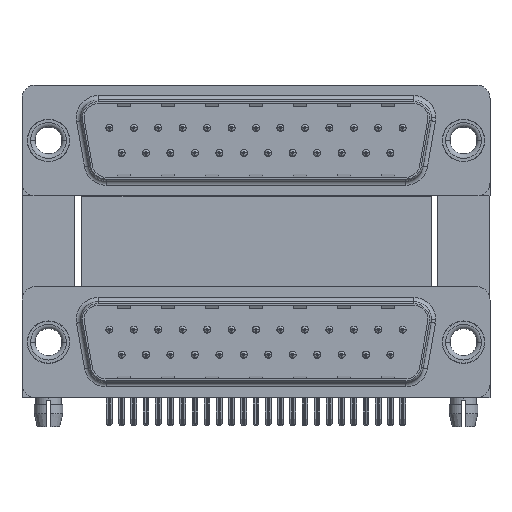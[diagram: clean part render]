
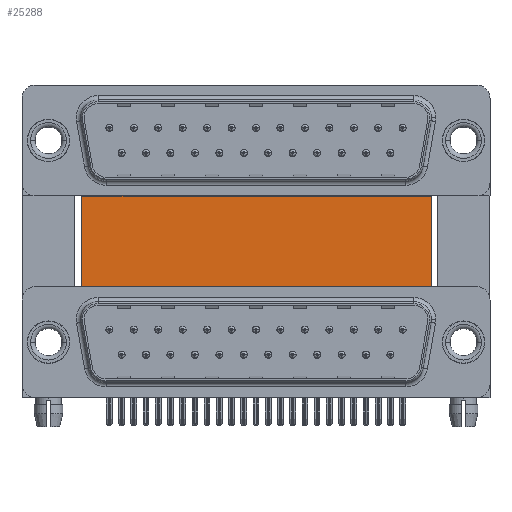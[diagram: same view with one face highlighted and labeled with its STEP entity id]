
A CAD part, top view. The second image highlights one B-rep face of the part: STEP entity #25288.
In plain terms, the highlighted planar face has unit normal (0, 0, 1).
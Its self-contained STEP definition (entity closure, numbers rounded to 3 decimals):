
#227 = CARTESIAN_POINT ( 'NONE',  ( 43.43, -3.735, -12. ) ) ;
#387 = LINE ( 'NONE', #34489, #16132 ) ;
#390 = CARTESIAN_POINT ( 'NONE',  ( 3.79, -3.735, -12. ) ) ;
#524 = DIRECTION ( 'NONE',  ( 0., 0., -1. ) ) ;
#559 = AXIS2_PLACEMENT_3D ( 'NONE', #4850, #524, #31419 ) ;
#2048 = EDGE_CURVE ( 'NONE', #22278, #27632, #387, .T. ) ;
#2146 = LINE ( 'NONE', #5746, #5574 ) ;
#3292 = ORIENTED_EDGE ( 'NONE', *, *, #9034, .F. ) ;
#4780 = VERTEX_POINT ( 'NONE', #227 ) ;
#4850 = CARTESIAN_POINT ( 'NONE',  ( 3.79, 16.585, -12. ) ) ;
#5574 = VECTOR ( 'NONE', #23992, 1000. ) ;
#5746 = CARTESIAN_POINT ( 'NONE',  ( 43.43, 16.585, -12. ) ) ;
#7857 = FACE_OUTER_BOUND ( 'NONE', #8169, .T. ) ;
#8169 = EDGE_LOOP ( 'NONE', ( #8323, #17312, #3292, #37066 ) ) ;
#8323 = ORIENTED_EDGE ( 'NONE', *, *, #10238, .T. ) ;
#9034 = EDGE_CURVE ( 'NONE', #22278, #30290, #38015, .T. ) ;
#9635 = DIRECTION ( 'NONE',  ( 0., -1., 0. ) ) ;
#10238 = EDGE_CURVE ( 'NONE', #27632, #4780, #27786, .T. ) ;
#15723 = CARTESIAN_POINT ( 'NONE',  ( 43.43, 16.585, -12. ) ) ;
#16132 = VECTOR ( 'NONE', #9635, 1000. ) ;
#16163 = DIRECTION ( 'NONE',  ( 1., 0., 0. ) ) ;
#17312 = ORIENTED_EDGE ( 'NONE', *, *, #29713, .F. ) ;
#20093 = PLANE ( 'NONE',  #559 ) ;
#22278 = VERTEX_POINT ( 'NONE', #27986 ) ;
#22373 = CARTESIAN_POINT ( 'NONE',  ( 3.79, -3.735, -12. ) ) ;
#23229 = VECTOR ( 'NONE', #23361, 1000. ) ;
#23361 = DIRECTION ( 'NONE',  ( 1., 0., 0. ) ) ;
#23992 = DIRECTION ( 'NONE',  ( 0., -1., 0. ) ) ;
#25288 = ADVANCED_FACE ( 'NONE', ( #7857 ), #20093, .F. ) ;
#25647 = VECTOR ( 'NONE', #16163, 1000. ) ;
#27632 = VERTEX_POINT ( 'NONE', #390 ) ;
#27786 = LINE ( 'NONE', #22373, #25647 ) ;
#27986 = CARTESIAN_POINT ( 'NONE',  ( 3.79, 16.585, -12. ) ) ;
#29713 = EDGE_CURVE ( 'NONE', #30290, #4780, #2146, .T. ) ;
#30290 = VERTEX_POINT ( 'NONE', #15723 ) ;
#31419 = DIRECTION ( 'NONE',  ( -1., 0., 0. ) ) ;
#34489 = CARTESIAN_POINT ( 'NONE',  ( 3.79, 16.585, -12. ) ) ;
#34804 = CARTESIAN_POINT ( 'NONE',  ( 3.79, 16.585, -12. ) ) ;
#37066 = ORIENTED_EDGE ( 'NONE', *, *, #2048, .T. ) ;
#38015 = LINE ( 'NONE', #34804, #23229 ) ;
